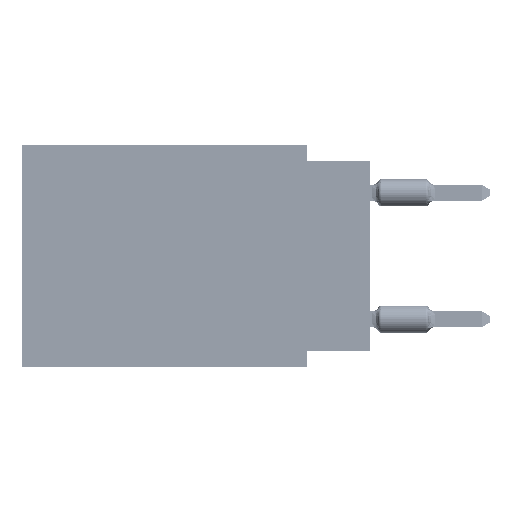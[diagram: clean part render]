
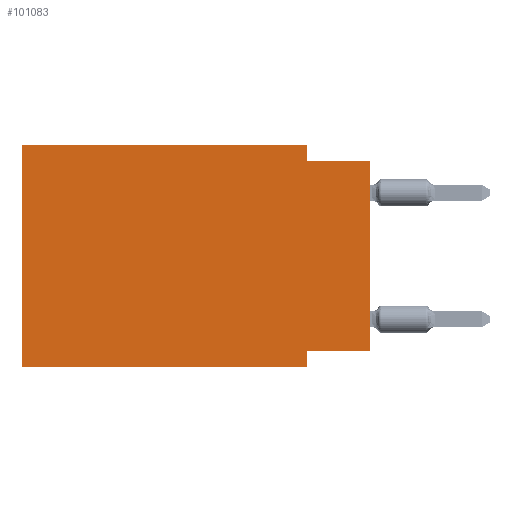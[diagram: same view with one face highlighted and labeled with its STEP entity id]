
A CAD part, left-side view. The second image highlights one B-rep face of the part: STEP entity #101083.
In plain terms, the highlighted planar face has unit normal (-1, 0, 0).
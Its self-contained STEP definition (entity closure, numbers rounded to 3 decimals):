
#43 = VECTOR ( 'NONE', #27813, 1000. ) ;
#1538 = EDGE_CURVE ( 'NONE', #105852, #37111, #32378, .T. ) ;
#5155 = CARTESIAN_POINT ( 'NONE',  ( 0., 0., 0. ) ) ;
#5511 = VECTOR ( 'NONE', #90372, 1000. ) ;
#8677 = EDGE_CURVE ( 'NONE', #97984, #39382, #46083, .T. ) ;
#9731 = ORIENTED_EDGE ( 'NONE', *, *, #34489, .F. ) ;
#10600 = DIRECTION ( 'NONE',  ( 0., -1., 0. ) ) ;
#13373 = VERTEX_POINT ( 'NONE', #26706 ) ;
#14536 = EDGE_CURVE ( 'NONE', #37111, #39940, #37107, .T. ) ;
#14922 = CARTESIAN_POINT ( 'NONE',  ( 0., 13.97, 0. ) ) ;
#15014 = ORIENTED_EDGE ( 'NONE', *, *, #81262, .F. ) ;
#16804 = VECTOR ( 'NONE', #96393, 1000. ) ;
#17431 = DIRECTION ( 'NONE',  ( 0., 0., -1. ) ) ;
#19236 = ORIENTED_EDGE ( 'NONE', *, *, #1538, .F. ) ;
#20123 = EDGE_CURVE ( 'NONE', #105852, #13373, #54194, .T. ) ;
#23337 = CARTESIAN_POINT ( 'NONE',  ( 0., 2.54, 0. ) ) ;
#24576 = AXIS2_PLACEMENT_3D ( 'NONE', #83344, #84424, #42452 ) ;
#24828 = ORIENTED_EDGE ( 'NONE', *, *, #20123, .T. ) ;
#25084 = CARTESIAN_POINT ( 'NONE',  ( 0., 2.54, -8.89 ) ) ;
#26706 = CARTESIAN_POINT ( 'NONE',  ( 0., 2.54, -8.89 ) ) ;
#26874 = CARTESIAN_POINT ( 'NONE',  ( 0., 2.54, -0.635 ) ) ;
#27662 = CARTESIAN_POINT ( 'NONE',  ( 0., 13.97, 0. ) ) ;
#27813 = DIRECTION ( 'NONE',  ( 0., -1., 0. ) ) ;
#32378 = LINE ( 'NONE', #14922, #94783 ) ;
#34489 = EDGE_CURVE ( 'NONE', #39940, #47812, #65838, .T. ) ;
#36645 = ORIENTED_EDGE ( 'NONE', *, *, #8677, .T. ) ;
#37107 = LINE ( 'NONE', #87262, #93529 ) ;
#37111 = VERTEX_POINT ( 'NONE', #27662 ) ;
#39382 = VERTEX_POINT ( 'NONE', #58657 ) ;
#39940 = VERTEX_POINT ( 'NONE', #92853 ) ;
#42452 = DIRECTION ( 'NONE',  ( 0., 0., -1. ) ) ;
#46083 = LINE ( 'NONE', #5155, #82134 ) ;
#46231 = LINE ( 'NONE', #72374, #16804 ) ;
#47812 = VERTEX_POINT ( 'NONE', #26874 ) ;
#54194 = LINE ( 'NONE', #77135, #57073 ) ;
#55827 = ORIENTED_EDGE ( 'NONE', *, *, #70000, .F. ) ;
#57073 = VECTOR ( 'NONE', #10600, 1000. ) ;
#57466 = VECTOR ( 'NONE', #17431, 1000. ) ;
#58657 = CARTESIAN_POINT ( 'NONE',  ( 0., 0., -0.635 ) ) ;
#62174 = DIRECTION ( 'NONE',  ( 0., -1., 0. ) ) ;
#65838 = LINE ( 'NONE', #23337, #5511 ) ;
#66402 = CARTESIAN_POINT ( 'NONE',  ( 0., 0., -8.255 ) ) ;
#66634 = VERTEX_POINT ( 'NONE', #74569 ) ;
#69249 = LINE ( 'NONE', #102506, #43 ) ;
#70000 = EDGE_CURVE ( 'NONE', #97984, #66634, #46231, .T. ) ;
#72374 = CARTESIAN_POINT ( 'NONE',  ( 0., 0., -8.255 ) ) ;
#74158 = LINE ( 'NONE', #25084, #57466 ) ;
#74346 = DIRECTION ( 'NONE',  ( 0., 0., 1. ) ) ;
#74569 = CARTESIAN_POINT ( 'NONE',  ( 0., 2.54, -8.255 ) ) ;
#76020 = EDGE_CURVE ( 'NONE', #47812, #39382, #69249, .T. ) ;
#77135 = CARTESIAN_POINT ( 'NONE',  ( 0., 13.97, -8.89 ) ) ;
#81262 = EDGE_CURVE ( 'NONE', #66634, #13373, #74158, .T. ) ;
#82134 = VECTOR ( 'NONE', #98376, 1000. ) ;
#82808 = FACE_OUTER_BOUND ( 'NONE', #85793, .T. ) ;
#83344 = CARTESIAN_POINT ( 'NONE',  ( 0., 13.97, 0. ) ) ;
#83704 = CARTESIAN_POINT ( 'NONE',  ( 0., 13.97, -8.89 ) ) ;
#84424 = DIRECTION ( 'NONE',  ( 1., 0., 0. ) ) ;
#85793 = EDGE_LOOP ( 'NONE', ( #36645, #86595, #9731, #106721, #19236, #24828, #15014, #55827 ) ) ;
#86595 = ORIENTED_EDGE ( 'NONE', *, *, #76020, .F. ) ;
#87262 = CARTESIAN_POINT ( 'NONE',  ( 0., 13.97, 0. ) ) ;
#90372 = DIRECTION ( 'NONE',  ( 0., 0., -1. ) ) ;
#92596 = PLANE ( 'NONE',  #24576 ) ;
#92853 = CARTESIAN_POINT ( 'NONE',  ( 0., 2.54, 0. ) ) ;
#93529 = VECTOR ( 'NONE', #62174, 1000. ) ;
#94783 = VECTOR ( 'NONE', #74346, 1000. ) ;
#96393 = DIRECTION ( 'NONE',  ( 0., 1., 0. ) ) ;
#97984 = VERTEX_POINT ( 'NONE', #66402 ) ;
#98376 = DIRECTION ( 'NONE',  ( 0., 0., 1. ) ) ;
#101083 = ADVANCED_FACE ( 'NONE', ( #82808 ), #92596, .F. ) ;
#102506 = CARTESIAN_POINT ( 'NONE',  ( 0., 0., -0.635 ) ) ;
#105852 = VERTEX_POINT ( 'NONE', #83704 ) ;
#106721 = ORIENTED_EDGE ( 'NONE', *, *, #14536, .F. ) ;
